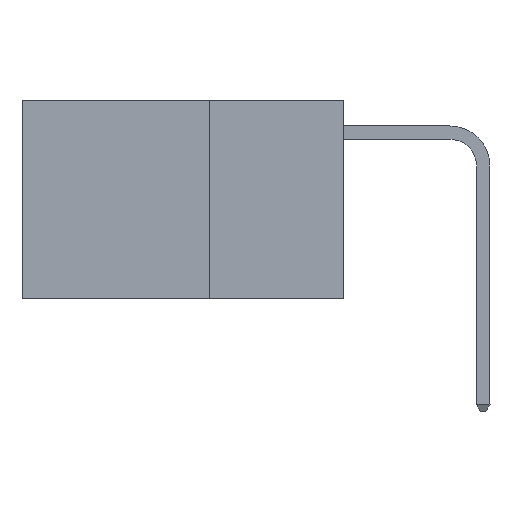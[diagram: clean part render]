
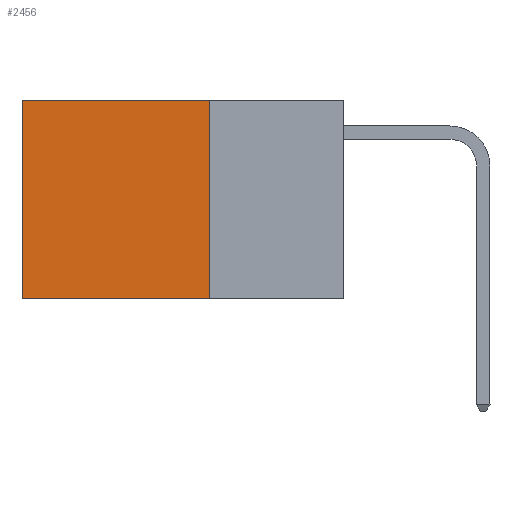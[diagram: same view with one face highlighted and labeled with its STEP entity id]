
A CAD part, left-side view. The second image highlights one B-rep face of the part: STEP entity #2456.
In plain terms, the highlighted planar face has unit normal (-1, 0, 0).
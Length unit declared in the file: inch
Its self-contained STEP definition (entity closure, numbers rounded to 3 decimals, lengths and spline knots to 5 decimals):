
#6 = LINE ( 'NONE', #12444, #11855 ) ;
#65 = CARTESIAN_POINT ( 'NONE',  ( 0.2625, 0.25, 0. ) ) ;
#417 = VECTOR ( 'NONE', #12825, 39.37008 ) ;
#1006 = LINE ( 'NONE', #9566, #9353 ) ;
#2019 = CARTESIAN_POINT ( 'NONE',  ( 0.2625, 0.25, 0. ) ) ;
#2048 = LINE ( 'NONE', #6928, #15491 ) ;
#2456 = ADVANCED_FACE ( 'NONE', ( #6146 ), #15825, .F. ) ;
#3479 = VERTEX_POINT ( 'NONE', #2019 ) ;
#3671 = EDGE_CURVE ( 'NONE', #3817, #15529, #6, .T. ) ;
#3817 = VERTEX_POINT ( 'NONE', #5589 ) ;
#5589 = CARTESIAN_POINT ( 'NONE',  ( 0.2625, 0.25, -0.37 ) ) ;
#5744 = AXIS2_PLACEMENT_3D ( 'NONE', #65, #14744, #8465 ) ;
#6146 = FACE_OUTER_BOUND ( 'NONE', #15331, .T. ) ;
#6928 = CARTESIAN_POINT ( 'NONE',  ( 0.2625, 0.6, 0. ) ) ;
#7355 = ORIENTED_EDGE ( 'NONE', *, *, #3671, .F. ) ;
#7826 = ORIENTED_EDGE ( 'NONE', *, *, #12952, .T. ) ;
#7905 = CARTESIAN_POINT ( 'NONE',  ( 0.2625, 0.25, 0. ) ) ;
#8465 = DIRECTION ( 'NONE',  ( 0., 0., -1. ) ) ;
#9353 = VECTOR ( 'NONE', #14096, 39.37008 ) ;
#9566 = CARTESIAN_POINT ( 'NONE',  ( 0.2625, 0.25, 0. ) ) ;
#10079 = LINE ( 'NONE', #7905, #417 ) ;
#10165 = CARTESIAN_POINT ( 'NONE',  ( 0.2625, 0.6, -0.37 ) ) ;
#10598 = EDGE_CURVE ( 'NONE', #11661, #15529, #2048, .T. ) ;
#11119 = CARTESIAN_POINT ( 'NONE',  ( 0.2625, 0.6, 0. ) ) ;
#11299 = DIRECTION ( 'NONE',  ( 0., 1., 0. ) ) ;
#11423 = ORIENTED_EDGE ( 'NONE', *, *, #10598, .T. ) ;
#11661 = VERTEX_POINT ( 'NONE', #11119 ) ;
#11855 = VECTOR ( 'NONE', #11299, 39.37008 ) ;
#12444 = CARTESIAN_POINT ( 'NONE',  ( 0.2625, 0.25, -0.37 ) ) ;
#12825 = DIRECTION ( 'NONE',  ( 0., 1., 0. ) ) ;
#12952 = EDGE_CURVE ( 'NONE', #3479, #11661, #10079, .T. ) ;
#13141 = EDGE_CURVE ( 'NONE', #3479, #3817, #1006, .T. ) ;
#13146 = ORIENTED_EDGE ( 'NONE', *, *, #13141, .F. ) ;
#13188 = DIRECTION ( 'NONE',  ( 0., 0., -1. ) ) ;
#14096 = DIRECTION ( 'NONE',  ( 0., 0., -1. ) ) ;
#14744 = DIRECTION ( 'NONE',  ( 1., 0., 0. ) ) ;
#15331 = EDGE_LOOP ( 'NONE', ( #11423, #7355, #13146, #7826 ) ) ;
#15491 = VECTOR ( 'NONE', #13188, 39.37008 ) ;
#15529 = VERTEX_POINT ( 'NONE', #10165 ) ;
#15825 = PLANE ( 'NONE',  #5744 ) ;
